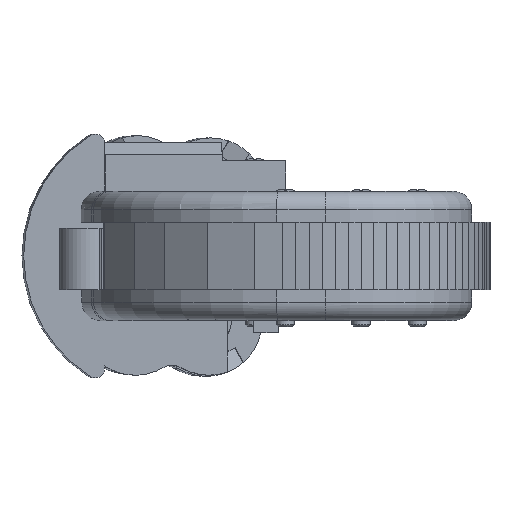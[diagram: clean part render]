
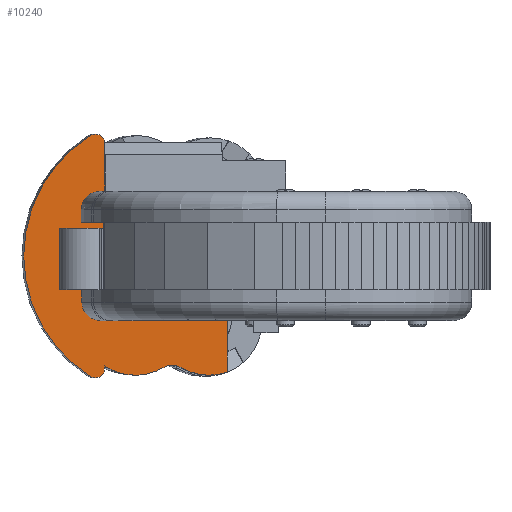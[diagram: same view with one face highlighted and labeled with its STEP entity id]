
A CAD part, left-side view. The second image highlights one B-rep face of the part: STEP entity #10240.
In plain terms, the highlighted face is planar.
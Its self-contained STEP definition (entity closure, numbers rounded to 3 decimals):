
#9514=CARTESIAN_POINT('',(-5.5,-31.024,0.0));
#9515=VERTEX_POINT('',#9514);
#9522=CARTESIAN_POINT('',(5.5,-31.024,0.0));
#9523=VERTEX_POINT('',#9522);
#9524=CARTESIAN_POINT('',(0.,-23.9,0.0));
#9525=DIRECTION('',(0.0,0.0,1.0));
#9526=DIRECTION('',(-0.611,-0.792,0.0));
#9527=AXIS2_PLACEMENT_3D('',#9524,#9525,#9526);
#9528=CIRCLE('',#9527,9.);
#9529=EDGE_CURVE('',#9515,#9523,#9528,.T.);
#9554=CARTESIAN_POINT('',(1.5,4.426,0.0));
#9555=VERTEX_POINT('',#9554);
#9556=CARTESIAN_POINT('',(-1.5,4.426,0.0));
#9557=VERTEX_POINT('',#9556);
#9558=CARTESIAN_POINT('',(1.5,4.426,0.0));
#9559=DIRECTION('',(-1.0,0.0,0.0));
#9560=VECTOR('',#9559,3.0);
#9561=LINE('',#9558,#9560);
#9562=EDGE_CURVE('',#9555,#9557,#9561,.T.);
#9594=CARTESIAN_POINT('',(1.5,-4.532,0.0));
#9595=VERTEX_POINT('',#9594);
#9596=CARTESIAN_POINT('',(1.5,-4.532,0.0));
#9597=DIRECTION('',(0.0,1.0,0.0));
#9598=VECTOR('',#9597,8.958);
#9599=LINE('',#9596,#9598);
#9600=EDGE_CURVE('',#9595,#9555,#9599,.T.);
#9625=CARTESIAN_POINT('',(-1.5,-4.532,0.0));
#9626=VERTEX_POINT('',#9625);
#9627=CARTESIAN_POINT('',(-1.5,-4.532,0.0));
#9628=DIRECTION('',(1.0,0.0,0.0));
#9629=VECTOR('',#9628,3.);
#9630=LINE('',#9627,#9629);
#9631=EDGE_CURVE('',#9626,#9595,#9630,.T.);
#9656=CARTESIAN_POINT('',(-1.5,4.426,0.0));
#9657=DIRECTION('',(0.0,-1.0,0.0));
#9658=VECTOR('',#9657,8.958);
#9659=LINE('',#9656,#9658);
#9660=EDGE_CURVE('',#9557,#9626,#9659,.T.);
#9689=CARTESIAN_POINT('',(2.0,-11.997,0.0));
#9690=VERTEX_POINT('',#9689);
#9691=CARTESIAN_POINT('',(0.0,-11.997,0.0));
#9692=DIRECTION('',(0.0,0.0,1.0));
#9693=DIRECTION('',(-1.0,0.0,0.0));
#9694=AXIS2_PLACEMENT_3D('',#9691,#9692,#9693);
#9695=CIRCLE('',#9694,2.0);
#9696=EDGE_CURVE('',#9690,#9690,#9695,.T.);
#9706=CARTESIAN_POINT('',(5.5,-20.9,0.0));
#9707=VERTEX_POINT('',#9706);
#9708=CARTESIAN_POINT('',(18.878,-20.9,0.0));
#9709=VERTEX_POINT('',#9708);
#9710=CARTESIAN_POINT('',(5.5,-20.9,0.0));
#9711=DIRECTION('',(1.0,0.0,0.0));
#9712=VECTOR('',#9711,13.378);
#9713=LINE('',#9710,#9712);
#9714=EDGE_CURVE('',#9707,#9709,#9713,.T.);
#9746=CARTESIAN_POINT('',(5.5,-31.024,0.0));
#9747=DIRECTION('',(0.0,1.0,0.0));
#9748=VECTOR('',#9747,10.124);
#9749=LINE('',#9746,#9748);
#9750=EDGE_CURVE('',#9523,#9707,#9749,.T.);
#9771=CARTESIAN_POINT('',(-5.5,-20.9,0.0));
#9772=VERTEX_POINT('',#9771);
#9773=CARTESIAN_POINT('',(-5.5,-20.9,0.0));
#9774=DIRECTION('',(0.0,-1.0,0.0));
#9775=VECTOR('',#9774,10.124);
#9776=LINE('',#9773,#9775);
#9777=EDGE_CURVE('',#9772,#9515,#9776,.T.);
#9805=CARTESIAN_POINT('',(-10.5,-20.9,0.0));
#9806=VERTEX_POINT('',#9805);
#9807=CARTESIAN_POINT('',(-10.5,-20.9,0.0));
#9808=DIRECTION('',(1.0,0.0,0.0));
#9809=VECTOR('',#9808,5.);
#9810=LINE('',#9807,#9809);
#9811=EDGE_CURVE('',#9806,#9772,#9810,.T.);
#9836=CARTESIAN_POINT('',(-10.5,-10.9,0.0));
#9837=VERTEX_POINT('',#9836);
#9838=CARTESIAN_POINT('',(-10.5,-10.9,0.0));
#9839=DIRECTION('',(0.0,-1.0,0.0));
#9840=VECTOR('',#9839,10.);
#9841=LINE('',#9838,#9840);
#9842=EDGE_CURVE('',#9837,#9806,#9841,.T.);
#9867=CARTESIAN_POINT('',(-10.392,-10.9,0.0));
#9868=VERTEX_POINT('',#9867);
#9869=CARTESIAN_POINT('',(-10.392,-10.9,0.0));
#9870=DIRECTION('',(-1.0,0.0,0.0));
#9871=VECTOR('',#9870,0.108);
#9872=LINE('',#9869,#9871);
#9873=EDGE_CURVE('',#9868,#9837,#9872,.T.);
#9898=CARTESIAN_POINT('',(-10.392,-0.9,0.0));
#9899=VERTEX_POINT('',#9898);
#9900=CARTESIAN_POINT('',(-10.392,-5.9,0.0));
#9901=DIRECTION('',(0.0,0.0,-1.0));
#9902=DIRECTION('',(0.0,1.0,0.0));
#9903=AXIS2_PLACEMENT_3D('',#9900,#9901,#9902);
#9904=CIRCLE('',#9903,5.);
#9905=EDGE_CURVE('',#9899,#9868,#9904,.T.);
#9931=CARTESIAN_POINT('',(-18.34,-0.9,0.0));
#9932=VERTEX_POINT('',#9931);
#9933=CARTESIAN_POINT('',(-18.34,-0.9,0.0));
#9934=DIRECTION('',(1.0,0.0,0.0));
#9935=VECTOR('',#9934,7.948);
#9936=LINE('',#9933,#9935);
#9937=EDGE_CURVE('',#9932,#9899,#9936,.T.);
#9962=CARTESIAN_POINT('',(-19.611,1.397,0.0));
#9963=VERTEX_POINT('',#9962);
#9964=CARTESIAN_POINT('',(-18.34,0.6,0.0));
#9965=DIRECTION('',(0.0,0.0,1.0));
#9966=DIRECTION('',(-0.847,0.531,0.0));
#9967=AXIS2_PLACEMENT_3D('',#9964,#9965,#9966);
#9968=CIRCLE('',#9967,1.5);
#9969=EDGE_CURVE('',#9963,#9932,#9968,.T.);
#9995=CARTESIAN_POINT('',(19.611,1.397,0.0));
#9996=VERTEX_POINT('',#9995);
#9997=CARTESIAN_POINT('',(0.,-10.9,0.0));
#9998=DIRECTION('',(0.0,0.0,1.0));
#9999=DIRECTION('',(0.847,0.531,0.0));
#10000=AXIS2_PLACEMENT_3D('',#9997,#9998,#9999);
#10001=CIRCLE('',#10000,23.147);
#10002=EDGE_CURVE('',#9996,#9963,#10001,.T.);
#10020=CARTESIAN_POINT('',(18.34,-0.9,0.0));
#10021=VERTEX_POINT('',#10020);
#10022=CARTESIAN_POINT('',(18.34,0.6,0.0));
#10023=DIRECTION('',(0.0,0.0,1.0));
#10024=DIRECTION('',(0.0,-1.0,0.0));
#10025=AXIS2_PLACEMENT_3D('',#10022,#10023,#10024);
#10026=CIRCLE('',#10025,1.5);
#10027=EDGE_CURVE('',#10021,#9996,#10026,.T.);
#10055=CARTESIAN_POINT('',(17.876,-0.9,0.0));
#10056=VERTEX_POINT('',#10055);
#10057=CARTESIAN_POINT('',(17.876,-0.9,0.0));
#10058=DIRECTION('',(1.0,0.0,0.0));
#10059=VECTOR('',#10058,0.464);
#10060=LINE('',#10057,#10059);
#10061=EDGE_CURVE('',#10056,#10021,#10060,.T.);
#10086=CARTESIAN_POINT('',(18.187,-10.4,0.0));
#10087=VERTEX_POINT('',#10086);
#10088=CARTESIAN_POINT('',(10.392,-5.9,0.0));
#10089=DIRECTION('',(0.0,0.0,1.0));
#10090=DIRECTION('',(0.866,-0.5,0.0));
#10091=AXIS2_PLACEMENT_3D('',#10088,#10089,#10090);
#10092=CIRCLE('',#10091,9.0);
#10093=EDGE_CURVE('',#10087,#10056,#10092,.T.);
#10119=CARTESIAN_POINT('',(18.187,-13.4,0.0));
#10120=VERTEX_POINT('',#10119);
#10121=CARTESIAN_POINT('',(20.785,-11.9,0.0));
#10122=DIRECTION('',(0.0,0.0,-1.0));
#10123=DIRECTION('',(0.866,-0.5,0.0));
#10124=AXIS2_PLACEMENT_3D('',#10121,#10122,#10123);
#10125=CIRCLE('',#10124,3.);
#10126=EDGE_CURVE('',#10120,#10087,#10125,.T.);
#10152=CARTESIAN_POINT('',(10.392,-17.9,0.0));
#10153=DIRECTION('',(0.0,0.0,1.0));
#10154=DIRECTION('',(0.943,-0.333,0.0));
#10155=AXIS2_PLACEMENT_3D('',#10152,#10153,#10154);
#10156=CIRCLE('',#10155,9.0);
#10157=EDGE_CURVE('',#9709,#10120,#10156,.T.);
#10208=CARTESIAN_POINT('',(0.913,-9.783,0.0));
#10209=DIRECTION('',(0.0,0.0,1.0));
#10210=DIRECTION('',(1.0,0.0,0.0));
#10211=AXIS2_PLACEMENT_3D('',#10208,#10209,#10210);
#10212=PLANE('',#10211);
#10213=ORIENTED_EDGE('',*,*,#10157,.F.);
#10214=ORIENTED_EDGE('',*,*,#9714,.F.);
#10215=ORIENTED_EDGE('',*,*,#9750,.F.);
#10216=ORIENTED_EDGE('',*,*,#9529,.F.);
#10217=ORIENTED_EDGE('',*,*,#9777,.F.);
#10218=ORIENTED_EDGE('',*,*,#9811,.F.);
#10219=ORIENTED_EDGE('',*,*,#9842,.F.);
#10220=ORIENTED_EDGE('',*,*,#9873,.F.);
#10221=ORIENTED_EDGE('',*,*,#9905,.F.);
#10222=ORIENTED_EDGE('',*,*,#9937,.F.);
#10223=ORIENTED_EDGE('',*,*,#9969,.F.);
#10224=ORIENTED_EDGE('',*,*,#10002,.F.);
#10225=ORIENTED_EDGE('',*,*,#10027,.F.);
#10226=ORIENTED_EDGE('',*,*,#10061,.F.);
#10227=ORIENTED_EDGE('',*,*,#10093,.F.);
#10228=ORIENTED_EDGE('',*,*,#10126,.F.);
#10229=EDGE_LOOP('',(#10213,#10214,#10215,#10216,#10217,#10218,#10219,#10220,#10221,#10222,#10223,#10224,#10225,#10226,#10227,#10228));
#10230=FACE_OUTER_BOUND('',#10229,.T.);
#10231=ORIENTED_EDGE('',*,*,#9562,.T.);
#10232=ORIENTED_EDGE('',*,*,#9660,.T.);
#10233=ORIENTED_EDGE('',*,*,#9631,.T.);
#10234=ORIENTED_EDGE('',*,*,#9600,.T.);
#10235=EDGE_LOOP('',(#10231,#10232,#10233,#10234));
#10236=FACE_BOUND('',#10235,.T.);
#10237=ORIENTED_EDGE('',*,*,#9696,.T.);
#10238=EDGE_LOOP('',(#10237));
#10239=FACE_BOUND('',#10238,.T.);
#10240=ADVANCED_FACE('',(#10230,#10236,#10239),#10212,.F.);
